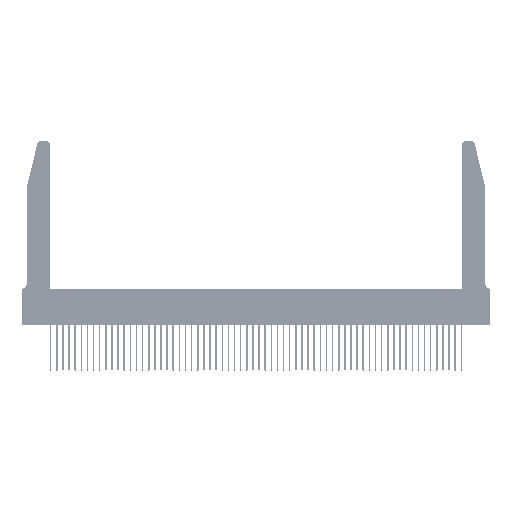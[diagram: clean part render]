
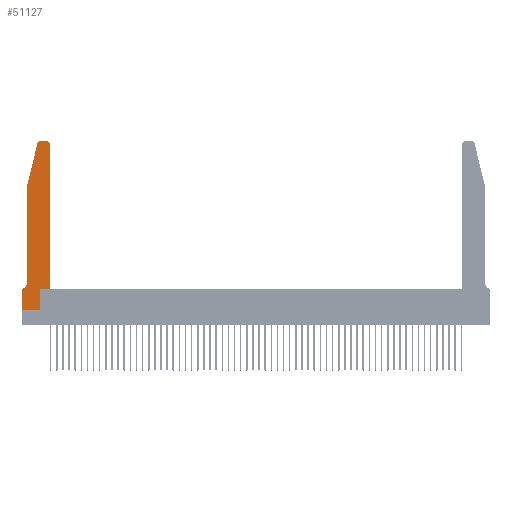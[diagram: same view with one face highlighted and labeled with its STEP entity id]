
A CAD part, top view. The second image highlights one B-rep face of the part: STEP entity #51127.
In plain terms, the highlighted planar face has unit normal (0, 0, 1).
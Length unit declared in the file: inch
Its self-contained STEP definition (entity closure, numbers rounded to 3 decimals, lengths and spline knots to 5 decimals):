
#389 = CARTESIAN_POINT ( 'NONE',  ( 0., 0., 0.37 ) ) ;
#849 = VECTOR ( 'NONE', #27238, 39.37008 ) ;
#884 = DIRECTION ( 'NONE',  ( 0., 0., 1. ) ) ;
#956 = CARTESIAN_POINT ( 'NONE',  ( 0.4505, 0.35, 0.37 ) ) ;
#1683 = VERTEX_POINT ( 'NONE', #40630 ) ;
#1900 = LINE ( 'NONE', #34144, #43430 ) ;
#1905 = DIRECTION ( 'NONE',  ( -1., 0., 0. ) ) ;
#2766 = ORIENTED_EDGE ( 'NONE', *, *, #9043, .T. ) ;
#3147 = VECTOR ( 'NONE', #47863, 39.37008 ) ;
#3533 = EDGE_LOOP ( 'NONE', ( #26984, #22871, #5067, #31582, #45297, #25265, #46152, #10935, #2766, #47191, #27994, #45598 ) ) ;
#5067 = ORIENTED_EDGE ( 'NONE', *, *, #35130, .T. ) ;
#5111 = CARTESIAN_POINT ( 'NONE',  ( 0.4205, 2.72, 0.37 ) ) ;
#5787 = EDGE_CURVE ( 'NONE', #21482, #22224, #24842, .T. ) ;
#7826 = EDGE_CURVE ( 'NONE', #9410, #39968, #32548, .T. ) ;
#8383 = FACE_OUTER_BOUND ( 'NONE', #3533, .T. ) ;
#9043 = EDGE_CURVE ( 'NONE', #39968, #20432, #11262, .T. ) ;
#9410 = VERTEX_POINT ( 'NONE', #18297 ) ;
#9523 = EDGE_CURVE ( 'NONE', #1683, #44749, #27729, .T. ) ;
#10686 = AXIS2_PLACEMENT_3D ( 'NONE', #5111, #51584, #47007 ) ;
#10825 = VECTOR ( 'NONE', #34700, 39.37008 ) ;
#10935 = ORIENTED_EDGE ( 'NONE', *, *, #7826, .T. ) ;
#11262 = LINE ( 'NONE', #12271, #46247 ) ;
#12262 = EDGE_CURVE ( 'NONE', #22224, #9410, #44400, .T. ) ;
#12271 = CARTESIAN_POINT ( 'NONE',  ( 0.2865, 0.35, 0.37 ) ) ;
#13581 = CARTESIAN_POINT ( 'NONE',  ( 0.0055, 0.35, 0.37 ) ) ;
#14335 = AXIS2_PLACEMENT_3D ( 'NONE', #15857, #884, #49901 ) ;
#15262 = EDGE_CURVE ( 'NONE', #18051, #53572, #53326, .T. ) ;
#15561 = PLANE ( 'NONE',  #14335 ) ;
#15857 = CARTESIAN_POINT ( 'NONE',  ( 0., 0.35, 0.37 ) ) ;
#15866 = VECTOR ( 'NONE', #1905, 39.37008 ) ;
#16389 = CARTESIAN_POINT ( 'NONE',  ( 0.4505, 2.72, 0.37 ) ) ;
#16554 = EDGE_CURVE ( 'NONE', #53400, #1683, #33364, .T. ) ;
#17338 = EDGE_CURVE ( 'NONE', #20432, #43933, #27971, .T. ) ;
#18051 = VERTEX_POINT ( 'NONE', #22283 ) ;
#18297 = CARTESIAN_POINT ( 'NONE',  ( 0., 0., 0.37 ) ) ;
#18469 = CARTESIAN_POINT ( 'NONE',  ( 0., 0.35, 0.37 ) ) ;
#18915 = VECTOR ( 'NONE', #45128, 39.37008 ) ;
#20432 = VERTEX_POINT ( 'NONE', #39504 ) ;
#21482 = VERTEX_POINT ( 'NONE', #13581 ) ;
#21540 = DIRECTION ( 'NONE',  ( 1., 0., 0. ) ) ;
#22224 = VERTEX_POINT ( 'NONE', #18469 ) ;
#22283 = CARTESIAN_POINT ( 'NONE',  ( 0.0755, 2., 0.37 ) ) ;
#22619 = CARTESIAN_POINT ( 'NONE',  ( 0.0755, 0.42, 0.37 ) ) ;
#22871 = ORIENTED_EDGE ( 'NONE', *, *, #40277, .T. ) ;
#23338 = CARTESIAN_POINT ( 'NONE',  ( 0.0755, 0.35, 0.37 ) ) ;
#24842 = LINE ( 'NONE', #23338, #18915 ) ;
#25024 = DIRECTION ( 'NONE',  ( 0., 0., -1. ) ) ;
#25265 = ORIENTED_EDGE ( 'NONE', *, *, #5787, .T. ) ;
#25739 = VERTEX_POINT ( 'NONE', #45535 ) ;
#26984 = ORIENTED_EDGE ( 'NONE', *, *, #9523, .T. ) ;
#27238 = DIRECTION ( 'NONE',  ( 0., -1., 0. ) ) ;
#27729 = LINE ( 'NONE', #52990, #15866 ) ;
#27838 = AXIS2_PLACEMENT_3D ( 'NONE', #46075, #25024, #41450 ) ;
#27880 = EDGE_CURVE ( 'NONE', #43933, #53400, #1900, .T. ) ;
#27971 = LINE ( 'NONE', #956, #10825 ) ;
#27994 = ORIENTED_EDGE ( 'NONE', *, *, #27880, .T. ) ;
#29202 = AXIS2_PLACEMENT_3D ( 'NONE', #33938, #41842, #21540 ) ;
#29246 = DIRECTION ( 'NONE',  ( 0., 1., 0. ) ) ;
#31582 = ORIENTED_EDGE ( 'NONE', *, *, #15262, .T. ) ;
#32548 = LINE ( 'NONE', #389, #41777 ) ;
#33364 = CIRCLE ( 'NONE', #10686, 0.03 ) ;
#33938 = CARTESIAN_POINT ( 'NONE',  ( 0.284, 2.72, 0.37 ) ) ;
#34144 = CARTESIAN_POINT ( 'NONE',  ( 0.4505, 0.35, 0.37 ) ) ;
#34700 = DIRECTION ( 'NONE',  ( 1., 0., 0. ) ) ;
#35130 = EDGE_CURVE ( 'NONE', #25739, #18051, #40516, .T. ) ;
#35227 = CARTESIAN_POINT ( 'NONE',  ( 0.4505, 0.35, 0.37 ) ) ;
#36186 = CARTESIAN_POINT ( 'NONE',  ( 0.0755, 2., 0.37 ) ) ;
#36372 = CARTESIAN_POINT ( 'NONE',  ( 0.2865, 0., 0.37 ) ) ;
#36505 = CIRCLE ( 'NONE', #27838, 0.07 ) ;
#39504 = CARTESIAN_POINT ( 'NONE',  ( 0.2865, 0.35, 0.37 ) ) ;
#39968 = VERTEX_POINT ( 'NONE', #36372 ) ;
#40277 = EDGE_CURVE ( 'NONE', #44749, #25739, #43608, .T. ) ;
#40404 = DIRECTION ( 'NONE',  ( -0.239, -0.971, 0. ) ) ;
#40516 = LINE ( 'NONE', #36186, #47801 ) ;
#40630 = CARTESIAN_POINT ( 'NONE',  ( 0.4205, 2.75, 0.37 ) ) ;
#41450 = DIRECTION ( 'NONE',  ( -1., 0., 0. ) ) ;
#41777 = VECTOR ( 'NONE', #47067, 39.37008 ) ;
#41842 = DIRECTION ( 'NONE',  ( 0., 0., 1. ) ) ;
#43430 = VECTOR ( 'NONE', #47075, 39.37008 ) ;
#43582 = CARTESIAN_POINT ( 'NONE',  ( 0.0755, 2., 0.37 ) ) ;
#43608 = CIRCLE ( 'NONE', #29202, 0.03 ) ;
#43933 = VERTEX_POINT ( 'NONE', #35227 ) ;
#44400 = LINE ( 'NONE', #52513, #849 ) ;
#44749 = VERTEX_POINT ( 'NONE', #53222 ) ;
#45128 = DIRECTION ( 'NONE',  ( -1., 0., 0. ) ) ;
#45297 = ORIENTED_EDGE ( 'NONE', *, *, #53407, .T. ) ;
#45535 = CARTESIAN_POINT ( 'NONE',  ( 0.25487, 2.72718, 0.37 ) ) ;
#45598 = ORIENTED_EDGE ( 'NONE', *, *, #16554, .T. ) ;
#46075 = CARTESIAN_POINT ( 'NONE',  ( 0.0055, 0.42, 0.37 ) ) ;
#46152 = ORIENTED_EDGE ( 'NONE', *, *, #12262, .T. ) ;
#46247 = VECTOR ( 'NONE', #29246, 39.37008 ) ;
#47007 = DIRECTION ( 'NONE',  ( 1., 0., 0. ) ) ;
#47067 = DIRECTION ( 'NONE',  ( 1., 0., 0. ) ) ;
#47075 = DIRECTION ( 'NONE',  ( 0., 1., 0. ) ) ;
#47191 = ORIENTED_EDGE ( 'NONE', *, *, #17338, .T. ) ;
#47801 = VECTOR ( 'NONE', #40404, 39.37008 ) ;
#47863 = DIRECTION ( 'NONE',  ( 0., -1., 0. ) ) ;
#49901 = DIRECTION ( 'NONE',  ( 1., 0., 0. ) ) ;
#51127 = ADVANCED_FACE ( 'NONE', ( #8383 ), #15561, .T. ) ;
#51584 = DIRECTION ( 'NONE',  ( 0., 0., 1. ) ) ;
#52513 = CARTESIAN_POINT ( 'NONE',  ( 0., 0., 0.37 ) ) ;
#52990 = CARTESIAN_POINT ( 'NONE',  ( 0.2605, 2.75, 0.37 ) ) ;
#53222 = CARTESIAN_POINT ( 'NONE',  ( 0.284, 2.75, 0.37 ) ) ;
#53326 = LINE ( 'NONE', #43582, #3147 ) ;
#53400 = VERTEX_POINT ( 'NONE', #16389 ) ;
#53407 = EDGE_CURVE ( 'NONE', #53572, #21482, #36505, .T. ) ;
#53572 = VERTEX_POINT ( 'NONE', #22619 ) ;
